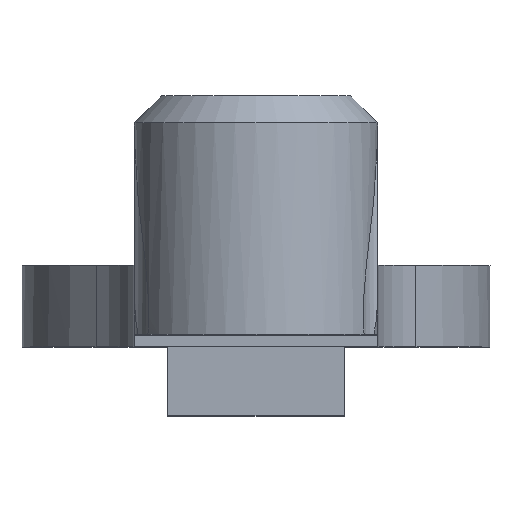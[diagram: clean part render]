
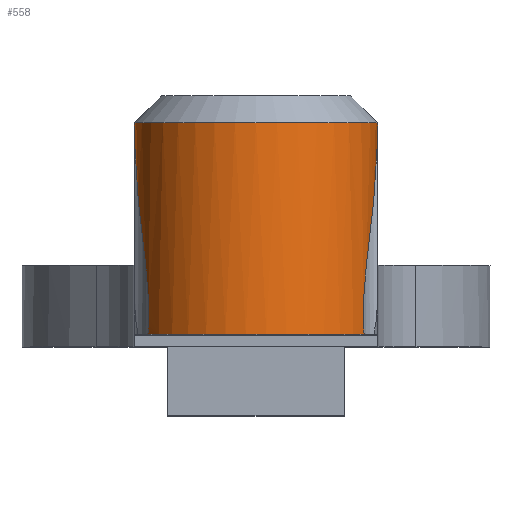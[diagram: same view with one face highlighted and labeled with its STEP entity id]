
A CAD part, top view. The second image highlights one B-rep face of the part: STEP entity #558.
In plain terms, the highlighted cylindrical face has radius 3.16 mm (diameter 6.32 mm), a partial arc.
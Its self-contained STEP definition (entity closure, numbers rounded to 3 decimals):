
#18 = VECTOR ( 'NONE', #1562, 1000. ) ;
#19 = LINE ( 'NONE', #1233, #22 ) ;
#22 = VECTOR ( 'NONE', #34, 1000. ) ;
#23 = CIRCLE ( 'NONE', #1823, 3.16 ) ;
#24 = LINE ( 'NONE', #40, #18 ) ;
#28 = CARTESIAN_POINT ( 'NONE',  ( 3.016, 5.155, 18.338 ) ) ;
#34 = DIRECTION ( 'NONE',  ( 0., -1., 0. ) ) ;
#40 = CARTESIAN_POINT ( 'NONE',  ( -3.16, 3.91, 17.385 ) ) ;
#48 = CARTESIAN_POINT ( 'NONE',  ( -3.065, 5.572, 18.175 ) ) ;
#68 = AXIS2_PLACEMENT_3D ( 'NONE', #1714, #724, #1812 ) ;
#187 = CARTESIAN_POINT ( 'NONE',  ( 2.864, 3.877, 18.724 ) ) ;
#205 = DIRECTION ( 'NONE',  ( 0., -1., 0. ) ) ;
#215 = CARTESIAN_POINT ( 'NONE',  ( -2.916, 4.307, 18.611 ) ) ;
#319 = CYLINDRICAL_SURFACE ( 'NONE', #1864, 3.16 ) ;
#337 = ORIENTED_EDGE ( 'NONE', *, *, #356, .F. ) ;
#356 = EDGE_CURVE ( 'NONE', #1515, #1094, #1632, .T. ) ;
#362 = EDGE_CURVE ( 'NONE', #1251, #1515, #19, .T. ) ;
#369 = CARTESIAN_POINT ( 'NONE',  ( 2.793, 2.989, 18.863 ) ) ;
#377 = EDGE_CURVE ( 'NONE', #1251, #1589, #23, .T. ) ;
#379 = EDGE_CURVE ( 'NONE', #1589, #1610, #24, .T. ) ;
#391 = EDGE_CURVE ( 'NONE', #1610, #1098, #1245, .T. ) ;
#392 = CARTESIAN_POINT ( 'NONE',  ( -2.807, 3.21, 18.836 ) ) ;
#431 = ORIENTED_EDGE ( 'NONE', *, *, #379, .T. ) ;
#470 = DIRECTION ( 'NONE',  ( 0., 0., -1. ) ) ;
#548 = CARTESIAN_POINT ( 'NONE',  ( 2.784, 2.538, 18.88 ) ) ;
#558 = ADVANCED_FACE ( 'NONE', ( #1636 ), #319, .T. ) ;
#563 = CARTESIAN_POINT ( 'NONE',  ( -3.16, 6.787, 17.611 ) ) ;
#571 = CARTESIAN_POINT ( 'NONE',  ( -2.784, 2.648, 18.879 ) ) ;
#591 = CARTESIAN_POINT ( 'NONE',  ( -2.815, 2.09, 18.821 ) ) ;
#674 = CARTESIAN_POINT ( 'NONE',  ( 3.16, 7.178, 17.385 ) ) ;
#705 = CARTESIAN_POINT ( 'NONE',  ( 3.137, 6.391, 17.81 ) ) ;
#711 = CARTESIAN_POINT ( 'NONE',  ( 3.16, 6.79, 17.609 ) ) ;
#721 = CARTESIAN_POINT ( 'NONE',  ( 2.798, 2.198, 18.853 ) ) ;
#724 = DIRECTION ( 'NONE',  ( 0., -1., 0. ) ) ;
#738 = CARTESIAN_POINT ( 'NONE',  ( -3.16, 7.178, 17.385 ) ) ;
#745 = CARTESIAN_POINT ( 'NONE',  ( -2.791, 2.311, 18.866 ) ) ;
#877 = ORIENTED_EDGE ( 'NONE', *, *, #377, .T. ) ;
#884 = CARTESIAN_POINT ( 'NONE',  ( 3.16, 7.178, 17.385 ) ) ;
#919 = CARTESIAN_POINT ( 'NONE',  ( -2.815, 2.09, 18.821 ) ) ;
#969 = ORIENTED_EDGE ( 'NONE', *, *, #1724, .F. ) ;
#1058 = CARTESIAN_POINT ( 'NONE',  ( 3.065, 5.574, 18.175 ) ) ;
#1094 = VERTEX_POINT ( 'NONE', #1433 ) ;
#1098 = VERTEX_POINT ( 'NONE', #591 ) ;
#1208 = CARTESIAN_POINT ( 'NONE',  ( -3.16, 7.59, 17.385 ) ) ;
#1224 = CARTESIAN_POINT ( 'NONE',  ( 2.916, 4.307, 18.611 ) ) ;
#1233 = CARTESIAN_POINT ( 'NONE',  ( 3.16, 3.91, 17.385 ) ) ;
#1238 = CARTESIAN_POINT ( 'NONE',  ( 0., 7.59, 17.385 ) ) ;
#1245 = B_SPLINE_CURVE_WITH_KNOTS ( 'NONE', 3,
 ( #738, #563, #1922, #48, #1246, #215, #1412, #392, #1578, #571, #1728, #745, #1825, #919 ),
 .UNSPECIFIED., .F., .F.,
 ( 4, 2, 2, 2, 2, 2, 4 ),
 ( 0., 0.001, 0.003, 0.004, 0.005, 0.005, 0.005 ),
 .UNSPECIFIED. ) ;
#1246 = CARTESIAN_POINT ( 'NONE',  ( -3.017, 5.157, 18.337 ) ) ;
#1251 = VERTEX_POINT ( 'NONE', #1309 ) ;
#1261 = CIRCLE ( 'NONE', #68, 3.16 ) ;
#1278 = ORIENTED_EDGE ( 'NONE', *, *, #362, .F. ) ;
#1309 = CARTESIAN_POINT ( 'NONE',  ( 3.16, 7.59, 17.385 ) ) ;
#1369 = CARTESIAN_POINT ( 'NONE',  ( -3.16, 7.178, 17.385 ) ) ;
#1379 = ORIENTED_EDGE ( 'NONE', *, *, #391, .T. ) ;
#1388 = CARTESIAN_POINT ( 'NONE',  ( 2.808, 3.215, 18.835 ) ) ;
#1403 = DIRECTION ( 'NONE',  ( 0., 0., 1. ) ) ;
#1412 = CARTESIAN_POINT ( 'NONE',  ( -2.863, 3.872, 18.725 ) ) ;
#1433 = CARTESIAN_POINT ( 'NONE',  ( 2.815, 2.09, 18.821 ) ) ;
#1515 = VERTEX_POINT ( 'NONE', #674 ) ;
#1553 = CARTESIAN_POINT ( 'NONE',  ( 2.784, 2.651, 18.879 ) ) ;
#1562 = DIRECTION ( 'NONE',  ( 0., -1., 0. ) ) ;
#1578 = CARTESIAN_POINT ( 'NONE',  ( -2.793, 2.988, 18.864 ) ) ;
#1589 = VERTEX_POINT ( 'NONE', #1208 ) ;
#1610 = VERTEX_POINT ( 'NONE', #1369 ) ;
#1632 = B_SPLINE_CURVE_WITH_KNOTS ( 'NONE', 3,
 ( #884, #711, #705, #1058, #28, #1224, #187, #1388, #369, #1553, #548, #1712, #721, #1810 ),
 .UNSPECIFIED., .F., .F.,
 ( 4, 2, 2, 2, 2, 2, 4 ),
 ( 0.008, 0.009, 0.01, 0.012, 0.012, 0.013, 0.013 ),
 .UNSPECIFIED. ) ;
#1636 = FACE_OUTER_BOUND ( 'NONE', #1649, .T. ) ;
#1649 = EDGE_LOOP ( 'NONE', ( #337, #1278, #877, #431, #1379, #969 ) ) ;
#1712 = CARTESIAN_POINT ( 'NONE',  ( 2.791, 2.313, 18.867 ) ) ;
#1714 = CARTESIAN_POINT ( 'NONE',  ( 0., 2.09, 17.385 ) ) ;
#1724 = EDGE_CURVE ( 'NONE', #1094, #1098, #1261, .T. ) ;
#1728 = CARTESIAN_POINT ( 'NONE',  ( -2.784, 2.535, 18.88 ) ) ;
#1810 = CARTESIAN_POINT ( 'NONE',  ( 2.815, 2.09, 18.821 ) ) ;
#1812 = DIRECTION ( 'NONE',  ( 0., 0., -1. ) ) ;
#1823 = AXIS2_PLACEMENT_3D ( 'NONE', #1238, #205, #1403 ) ;
#1825 = CARTESIAN_POINT ( 'NONE',  ( -2.798, 2.199, 18.854 ) ) ;
#1861 = CARTESIAN_POINT ( 'NONE',  ( 0., 3.91, 17.385 ) ) ;
#1864 = AXIS2_PLACEMENT_3D ( 'NONE', #1861, #1959, #470 ) ;
#1922 = CARTESIAN_POINT ( 'NONE',  ( -3.136, 6.387, 17.812 ) ) ;
#1959 = DIRECTION ( 'NONE',  ( 0., -1., 0. ) ) ;
